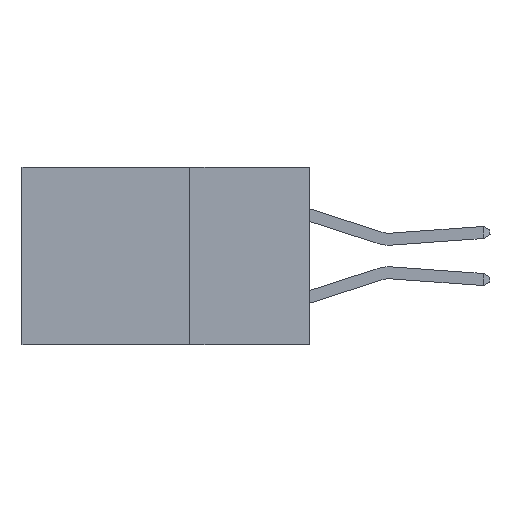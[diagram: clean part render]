
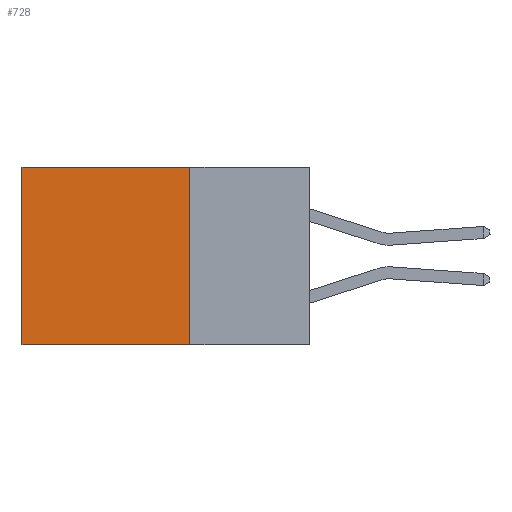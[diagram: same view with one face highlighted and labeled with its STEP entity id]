
A CAD part, left-side view. The second image highlights one B-rep face of the part: STEP entity #728.
In plain terms, the highlighted planar face has unit normal (-1, 0, 0).
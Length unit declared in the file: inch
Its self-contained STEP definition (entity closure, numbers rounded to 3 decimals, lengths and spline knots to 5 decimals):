
#188 = ORIENTED_EDGE ( 'NONE', *, *, #24243, .F. ) ;
#728 = ADVANCED_FACE ( 'NONE', ( #1364 ), #10648, .F. ) ;
#905 = EDGE_CURVE ( 'NONE', #2234, #23955, #13617, .T. ) ;
#1364 = FACE_OUTER_BOUND ( 'NONE', #20703, .T. ) ;
#1810 = ORIENTED_EDGE ( 'NONE', *, *, #26305, .T. ) ;
#1864 = ORIENTED_EDGE ( 'NONE', *, *, #15381, .T. ) ;
#2234 = VERTEX_POINT ( 'NONE', #16549 ) ;
#4238 = VECTOR ( 'NONE', #25582, 39.37008 ) ;
#4404 = VECTOR ( 'NONE', #5969, 39.37008 ) ;
#4940 = CARTESIAN_POINT ( 'NONE',  ( 0.298, 0.25, 0. ) ) ;
#5691 = ORIENTED_EDGE ( 'NONE', *, *, #905, .F. ) ;
#5969 = DIRECTION ( 'NONE',  ( 0., 0., -1. ) ) ;
#7999 = VECTOR ( 'NONE', #9243, 39.37008 ) ;
#9243 = DIRECTION ( 'NONE',  ( 0., 1., 0. ) ) ;
#10102 = CARTESIAN_POINT ( 'NONE',  ( 0.298, 0.6, 0. ) ) ;
#10402 = CARTESIAN_POINT ( 'NONE',  ( 0.298, 0.25, 0. ) ) ;
#10539 = CARTESIAN_POINT ( 'NONE',  ( 0.298, 0.25, -0.37 ) ) ;
#10648 = PLANE ( 'NONE',  #12479 ) ;
#12479 = AXIS2_PLACEMENT_3D ( 'NONE', #10402, #15804, #15299 ) ;
#12526 = VERTEX_POINT ( 'NONE', #17443 ) ;
#13617 = LINE ( 'NONE', #10539, #7999 ) ;
#15299 = DIRECTION ( 'NONE',  ( 0., 0., -1. ) ) ;
#15381 = EDGE_CURVE ( 'NONE', #12526, #23955, #15621, .T. ) ;
#15621 = LINE ( 'NONE', #10102, #4404 ) ;
#15804 = DIRECTION ( 'NONE',  ( 1., 0., 0. ) ) ;
#16549 = CARTESIAN_POINT ( 'NONE',  ( 0.298, 0.25, -0.37 ) ) ;
#16961 = LINE ( 'NONE', #4940, #23236 ) ;
#17443 = CARTESIAN_POINT ( 'NONE',  ( 0.298, 0.6, 0. ) ) ;
#19717 = DIRECTION ( 'NONE',  ( 0., 0., -1. ) ) ;
#20703 = EDGE_LOOP ( 'NONE', ( #1864, #5691, #188, #1810 ) ) ;
#21137 = LINE ( 'NONE', #23477, #4238 ) ;
#22919 = VERTEX_POINT ( 'NONE', #24229 ) ;
#23078 = CARTESIAN_POINT ( 'NONE',  ( 0.298, 0.6, -0.37 ) ) ;
#23236 = VECTOR ( 'NONE', #19717, 39.37008 ) ;
#23477 = CARTESIAN_POINT ( 'NONE',  ( 0.298, 0.25, 0. ) ) ;
#23955 = VERTEX_POINT ( 'NONE', #23078 ) ;
#24229 = CARTESIAN_POINT ( 'NONE',  ( 0.298, 0.25, 0. ) ) ;
#24243 = EDGE_CURVE ( 'NONE', #22919, #2234, #16961, .T. ) ;
#25582 = DIRECTION ( 'NONE',  ( 0., 1., 0. ) ) ;
#26305 = EDGE_CURVE ( 'NONE', #22919, #12526, #21137, .T. ) ;
